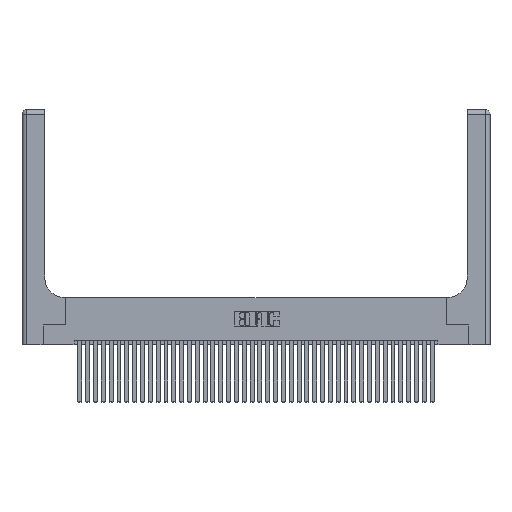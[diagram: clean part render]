
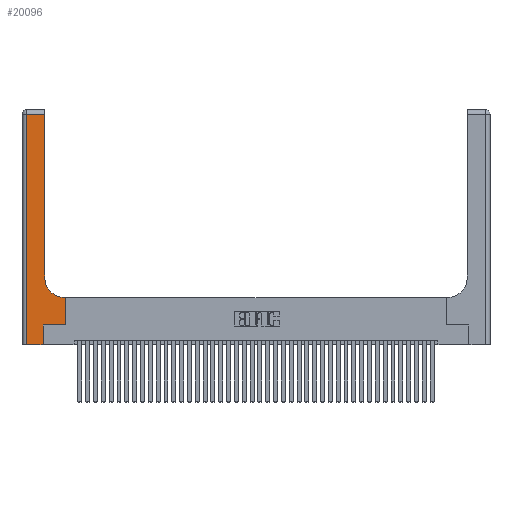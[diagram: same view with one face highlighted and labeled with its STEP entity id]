
A CAD part, top view. The second image highlights one B-rep face of the part: STEP entity #20096.
In plain terms, the highlighted planar face has unit normal (0, 0, 1).
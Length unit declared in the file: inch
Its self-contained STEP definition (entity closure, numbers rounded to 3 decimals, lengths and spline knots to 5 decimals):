
#342 = ORIENTED_EDGE ( 'NONE', *, *, #39798, .T. ) ;
#569 = ORIENTED_EDGE ( 'NONE', *, *, #21328, .T. ) ;
#698 = ORIENTED_EDGE ( 'NONE', *, *, #32670, .T. ) ;
#1017 = CARTESIAN_POINT ( 'NONE',  ( 0.5585, 0.25, 0.37 ) ) ;
#1382 = LINE ( 'NONE', #8026, #30863 ) ;
#2940 = AXIS2_PLACEMENT_3D ( 'NONE', #40577, #3027, #6145 ) ;
#3027 = DIRECTION ( 'NONE',  ( 0., 0., -1. ) ) ;
#3554 = LINE ( 'NONE', #34438, #26557 ) ;
#3857 = LINE ( 'NONE', #28664, #26357 ) ;
#3889 = FACE_OUTER_BOUND ( 'NONE', #5945, .T. ) ;
#3984 = LINE ( 'NONE', #29068, #5938 ) ;
#4366 = DIRECTION ( 'NONE',  ( 1., 0., 0. ) ) ;
#5587 = CARTESIAN_POINT ( 'NONE',  ( 0.269, 0., 0.37 ) ) ;
#5938 = VECTOR ( 'NONE', #4366, 39.37008 ) ;
#5945 = EDGE_LOOP ( 'NONE', ( #23842, #22899, #23359, #17495, #342, #698, #33870, #34570, #569 ) ) ;
#5993 = CARTESIAN_POINT ( 'NONE',  ( 0.269, 0.25, 0.37 ) ) ;
#6145 = DIRECTION ( 'NONE',  ( 1., 0., 0. ) ) ;
#7531 = VECTOR ( 'NONE', #11104, 39.37008 ) ;
#8026 = CARTESIAN_POINT ( 'NONE',  ( 0., 2.94, 0.37 ) ) ;
#9773 = EDGE_CURVE ( 'NONE', #25945, #14533, #31092, .T. ) ;
#9793 = DIRECTION ( 'NONE',  ( -1., 0., 0. ) ) ;
#11104 = DIRECTION ( 'NONE',  ( 1., 0., 0. ) ) ;
#11107 = DIRECTION ( 'NONE',  ( 0., -1., 0. ) ) ;
#11333 = CARTESIAN_POINT ( 'NONE',  ( 0.5585, 0.25, 0.37 ) ) ;
#12091 = CIRCLE ( 'NONE', #2940, 0.25 ) ;
#12885 = VERTEX_POINT ( 'NONE', #19284 ) ;
#13198 = DIRECTION ( 'NONE',  ( 0., 1., 0. ) ) ;
#14526 = CARTESIAN_POINT ( 'NONE',  ( 0.5585, 0.6, 0.37 ) ) ;
#14533 = VERTEX_POINT ( 'NONE', #27554 ) ;
#15079 = EDGE_CURVE ( 'NONE', #33421, #28459, #24704, .T. ) ;
#17495 = ORIENTED_EDGE ( 'NONE', *, *, #26866, .T. ) ;
#19110 = VERTEX_POINT ( 'NONE', #29754 ) ;
#19284 = CARTESIAN_POINT ( 'NONE',  ( 0.2915, 2.94, 0.37 ) ) ;
#19819 = VECTOR ( 'NONE', #20871, 39.37008 ) ;
#20087 = CARTESIAN_POINT ( 'NONE',  ( 0.269, 0.25, 0.37 ) ) ;
#20096 = ADVANCED_FACE ( 'NONE', ( #3889 ), #26638, .F. ) ;
#20212 = EDGE_CURVE ( 'NONE', #12885, #25945, #1382, .T. ) ;
#20266 = VECTOR ( 'NONE', #11107, 39.37008 ) ;
#20871 = DIRECTION ( 'NONE',  ( 0., 1., 0. ) ) ;
#21328 = EDGE_CURVE ( 'NONE', #22269, #19110, #12091, .T. ) ;
#22195 = EDGE_CURVE ( 'NONE', #28459, #22269, #3857, .T. ) ;
#22269 = VERTEX_POINT ( 'NONE', #38123 ) ;
#22637 = AXIS2_PLACEMENT_3D ( 'NONE', #39432, #23849, #36284 ) ;
#22899 = ORIENTED_EDGE ( 'NONE', *, *, #20212, .T. ) ;
#23359 = ORIENTED_EDGE ( 'NONE', *, *, #9773, .T. ) ;
#23574 = VERTEX_POINT ( 'NONE', #31453 ) ;
#23842 = ORIENTED_EDGE ( 'NONE', *, *, #34813, .T. ) ;
#23849 = DIRECTION ( 'NONE',  ( 0., 0., -1. ) ) ;
#24701 = DIRECTION ( 'NONE',  ( -1., 0., 0. ) ) ;
#24704 = LINE ( 'NONE', #1017, #32527 ) ;
#25945 = VERTEX_POINT ( 'NONE', #30155 ) ;
#26357 = VECTOR ( 'NONE', #24701, 39.37008 ) ;
#26557 = VECTOR ( 'NONE', #30893, 39.37008 ) ;
#26638 = PLANE ( 'NONE',  #22637 ) ;
#26743 = CARTESIAN_POINT ( 'NONE',  ( 0.06, 3., 0.37 ) ) ;
#26866 = EDGE_CURVE ( 'NONE', #14533, #23574, #3984, .T. ) ;
#27554 = CARTESIAN_POINT ( 'NONE',  ( 0.06, 0., 0.37 ) ) ;
#28225 = LINE ( 'NONE', #20087, #7531 ) ;
#28459 = VERTEX_POINT ( 'NONE', #14526 ) ;
#28664 = CARTESIAN_POINT ( 'NONE',  ( 0.2915, 0.6, 0.37 ) ) ;
#29068 = CARTESIAN_POINT ( 'NONE',  ( 0., 0., 0.37 ) ) ;
#29106 = VERTEX_POINT ( 'NONE', #5993 ) ;
#29754 = CARTESIAN_POINT ( 'NONE',  ( 0.2915, 0.85, 0.37 ) ) ;
#30155 = CARTESIAN_POINT ( 'NONE',  ( 0.06, 2.94, 0.37 ) ) ;
#30599 = LINE ( 'NONE', #5587, #19819 ) ;
#30863 = VECTOR ( 'NONE', #9793, 39.37008 ) ;
#30893 = DIRECTION ( 'NONE',  ( 0., 1., 0. ) ) ;
#31092 = LINE ( 'NONE', #26743, #20266 ) ;
#31453 = CARTESIAN_POINT ( 'NONE',  ( 0.269, 0., 0.37 ) ) ;
#32527 = VECTOR ( 'NONE', #13198, 39.37008 ) ;
#32670 = EDGE_CURVE ( 'NONE', #29106, #33421, #28225, .T. ) ;
#33421 = VERTEX_POINT ( 'NONE', #11333 ) ;
#33870 = ORIENTED_EDGE ( 'NONE', *, *, #15079, .T. ) ;
#34438 = CARTESIAN_POINT ( 'NONE',  ( 0.2915, 3., 0.37 ) ) ;
#34570 = ORIENTED_EDGE ( 'NONE', *, *, #22195, .T. ) ;
#34813 = EDGE_CURVE ( 'NONE', #19110, #12885, #3554, .T. ) ;
#36284 = DIRECTION ( 'NONE',  ( -1., 0., 0. ) ) ;
#38123 = CARTESIAN_POINT ( 'NONE',  ( 0.5415, 0.6, 0.37 ) ) ;
#39432 = CARTESIAN_POINT ( 'NONE',  ( 0., 3., 0.37 ) ) ;
#39798 = EDGE_CURVE ( 'NONE', #23574, #29106, #30599, .T. ) ;
#40577 = CARTESIAN_POINT ( 'NONE',  ( 0.5415, 0.85, 0.37 ) ) ;
